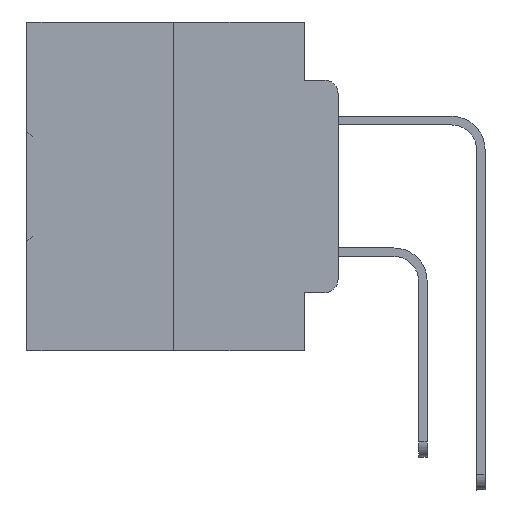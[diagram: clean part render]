
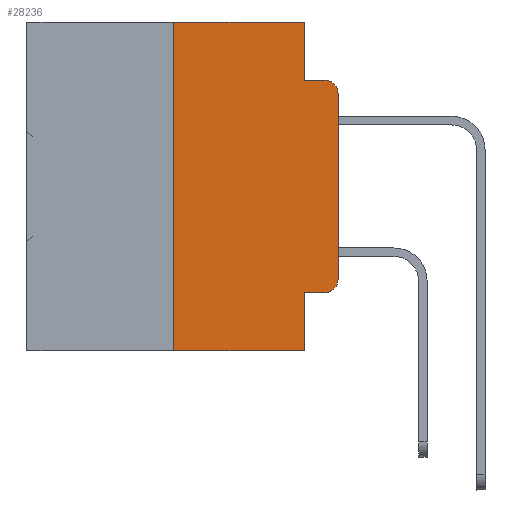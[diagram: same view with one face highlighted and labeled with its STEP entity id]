
A CAD part, left-side view. The second image highlights one B-rep face of the part: STEP entity #28236.
In plain terms, the highlighted planar face has unit normal (-1, 0, 0).
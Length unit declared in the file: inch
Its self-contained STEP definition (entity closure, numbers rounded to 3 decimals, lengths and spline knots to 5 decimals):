
#612 = LINE ( 'NONE', #32820, #22195 ) ;
#1276 = DIRECTION ( 'NONE',  ( 0., 0., -1. ) ) ;
#1624 = PLANE ( 'NONE',  #29660 ) ;
#1747 = DIRECTION ( 'NONE',  ( 0., 0., -1. ) ) ;
#1762 = VERTEX_POINT ( 'NONE', #13487 ) ;
#2349 = CARTESIAN_POINT ( 'NONE',  ( 0., 0.473, 0. ) ) ;
#2599 = LINE ( 'NONE', #25400, #31314 ) ;
#4646 = VERTEX_POINT ( 'NONE', #18591 ) ;
#5153 = LINE ( 'NONE', #27371, #21691 ) ;
#5428 = CARTESIAN_POINT ( 'NONE',  ( 0., 0.051, 0. ) ) ;
#6686 = AXIS2_PLACEMENT_3D ( 'NONE', #34584, #18198, #1276 ) ;
#6878 = VERTEX_POINT ( 'NONE', #7306 ) ;
#7306 = CARTESIAN_POINT ( 'NONE',  ( 0., 0.25, 0. ) ) ;
#7664 = ORIENTED_EDGE ( 'NONE', *, *, #12034, .F. ) ;
#7748 = CARTESIAN_POINT ( 'NONE',  ( 0., 0.051, -0.0885 ) ) ;
#9060 = VECTOR ( 'NONE', #16055, 39.37008 ) ;
#10329 = ORIENTED_EDGE ( 'NONE', *, *, #17287, .F. ) ;
#10410 = VECTOR ( 'NONE', #18750, 39.37008 ) ;
#10644 = FACE_OUTER_BOUND ( 'NONE', #27355, .T. ) ;
#10918 = DIRECTION ( 'NONE',  ( 0., -1., 0. ) ) ;
#11259 = LINE ( 'NONE', #7748, #10410 ) ;
#11261 = VERTEX_POINT ( 'NONE', #15993 ) ;
#11591 = ORIENTED_EDGE ( 'NONE', *, *, #33826, .T. ) ;
#12034 = EDGE_CURVE ( 'NONE', #6878, #1762, #16180, .T. ) ;
#12046 = ORIENTED_EDGE ( 'NONE', *, *, #13590, .T. ) ;
#13487 = CARTESIAN_POINT ( 'NONE',  ( 0., 0.051, 0. ) ) ;
#13590 = EDGE_CURVE ( 'NONE', #22594, #16457, #24282, .T. ) ;
#14485 = DIRECTION ( 'NONE',  ( 0., 0., 1. ) ) ;
#14914 = DIRECTION ( 'NONE',  ( 0., -1., 0. ) ) ;
#15206 = VERTEX_POINT ( 'NONE', #34273 ) ;
#15426 = EDGE_CURVE ( 'NONE', #15206, #22594, #5153, .T. ) ;
#15659 = CARTESIAN_POINT ( 'NONE',  ( 0., 0.02, -0.1085 ) ) ;
#15826 = CIRCLE ( 'NONE', #22721, 0.02 ) ;
#15993 = CARTESIAN_POINT ( 'NONE',  ( 0., 0.051, -0.5 ) ) ;
#16055 = DIRECTION ( 'NONE',  ( 0., 0., -1. ) ) ;
#16180 = LINE ( 'NONE', #2349, #24342 ) ;
#16457 = VERTEX_POINT ( 'NONE', #18059 ) ;
#17287 = EDGE_CURVE ( 'NONE', #15206, #11261, #29252, .T. ) ;
#17344 = CARTESIAN_POINT ( 'NONE',  ( 0., 0.02, -0.0885 ) ) ;
#18059 = CARTESIAN_POINT ( 'NONE',  ( 0., 0., -0.3915 ) ) ;
#18198 = DIRECTION ( 'NONE',  ( -1., 0., 0. ) ) ;
#18451 = DIRECTION ( 'NONE',  ( 0., 0., -1. ) ) ;
#18554 = LINE ( 'NONE', #34105, #32257 ) ;
#18591 = CARTESIAN_POINT ( 'NONE',  ( 0., 0., -0.1085 ) ) ;
#18638 = DIRECTION ( 'NONE',  ( 1., 0., 0. ) ) ;
#18750 = DIRECTION ( 'NONE',  ( 0., -1., 0. ) ) ;
#19747 = ORIENTED_EDGE ( 'NONE', *, *, #31977, .F. ) ;
#19943 = LINE ( 'NONE', #5428, #26381 ) ;
#20619 = ORIENTED_EDGE ( 'NONE', *, *, #26485, .F. ) ;
#21691 = VECTOR ( 'NONE', #10918, 39.37008 ) ;
#21972 = DIRECTION ( 'NONE',  ( 0., -1., 0. ) ) ;
#22195 = VECTOR ( 'NONE', #32947, 39.37008 ) ;
#22357 = ORIENTED_EDGE ( 'NONE', *, *, #24644, .F. ) ;
#22594 = VERTEX_POINT ( 'NONE', #28509 ) ;
#22721 = AXIS2_PLACEMENT_3D ( 'NONE', #15659, #34842, #18451 ) ;
#24282 = CIRCLE ( 'NONE', #6686, 0.02 ) ;
#24342 = VECTOR ( 'NONE', #21972, 39.37008 ) ;
#24644 = EDGE_CURVE ( 'NONE', #26163, #6878, #612, .T. ) ;
#24928 = CARTESIAN_POINT ( 'NONE',  ( 0., 0.051, -0.0885 ) ) ;
#25400 = CARTESIAN_POINT ( 'NONE',  ( 0., 0., 0. ) ) ;
#25766 = ORIENTED_EDGE ( 'NONE', *, *, #15426, .T. ) ;
#25769 = CARTESIAN_POINT ( 'NONE',  ( 0., 0.25, -0.5 ) ) ;
#26163 = VERTEX_POINT ( 'NONE', #25769 ) ;
#26381 = VECTOR ( 'NONE', #27592, 39.37008 ) ;
#26485 = EDGE_CURVE ( 'NONE', #1762, #26507, #19943, .T. ) ;
#26507 = VERTEX_POINT ( 'NONE', #24928 ) ;
#27355 = EDGE_LOOP ( 'NONE', ( #32605, #11591, #19747, #20619, #7664, #22357, #31344, #10329, #25766, #12046 ) ) ;
#27371 = CARTESIAN_POINT ( 'NONE',  ( 0., 0.051, -0.4115 ) ) ;
#27592 = DIRECTION ( 'NONE',  ( 0., 0., -1. ) ) ;
#28236 = ADVANCED_FACE ( 'NONE', ( #10644 ), #1624, .F. ) ;
#28509 = CARTESIAN_POINT ( 'NONE',  ( 0., 0.02, -0.4115 ) ) ;
#29252 = LINE ( 'NONE', #32483, #9060 ) ;
#29660 = AXIS2_PLACEMENT_3D ( 'NONE', #35033, #18638, #1747 ) ;
#31314 = VECTOR ( 'NONE', #14485, 39.37008 ) ;
#31344 = ORIENTED_EDGE ( 'NONE', *, *, #34276, .T. ) ;
#31977 = EDGE_CURVE ( 'NONE', #26507, #34199, #11259, .T. ) ;
#32257 = VECTOR ( 'NONE', #14914, 39.37008 ) ;
#32483 = CARTESIAN_POINT ( 'NONE',  ( 0., 0.051, 0. ) ) ;
#32605 = ORIENTED_EDGE ( 'NONE', *, *, #35637, .T. ) ;
#32820 = CARTESIAN_POINT ( 'NONE',  ( 0., 0.25, 0. ) ) ;
#32947 = DIRECTION ( 'NONE',  ( 0., 0., 1. ) ) ;
#33826 = EDGE_CURVE ( 'NONE', #4646, #34199, #15826, .T. ) ;
#34105 = CARTESIAN_POINT ( 'NONE',  ( 0., 0.473, -0.5 ) ) ;
#34199 = VERTEX_POINT ( 'NONE', #17344 ) ;
#34273 = CARTESIAN_POINT ( 'NONE',  ( 0., 0.051, -0.4115 ) ) ;
#34276 = EDGE_CURVE ( 'NONE', #26163, #11261, #18554, .T. ) ;
#34584 = CARTESIAN_POINT ( 'NONE',  ( 0., 0.02, -0.3915 ) ) ;
#34842 = DIRECTION ( 'NONE',  ( -1., 0., 0. ) ) ;
#35033 = CARTESIAN_POINT ( 'NONE',  ( 0., 0.473, 0. ) ) ;
#35637 = EDGE_CURVE ( 'NONE', #16457, #4646, #2599, .T. ) ;
